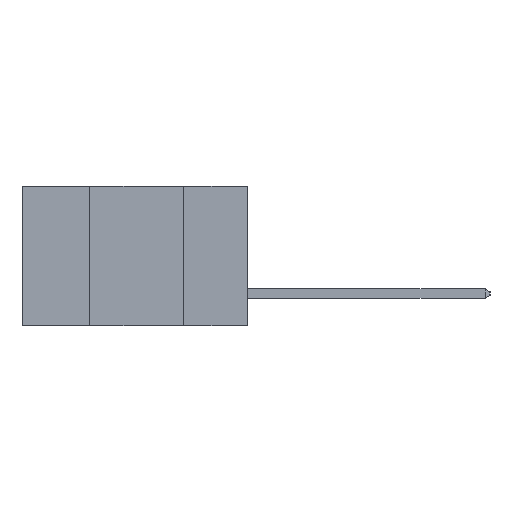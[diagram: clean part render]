
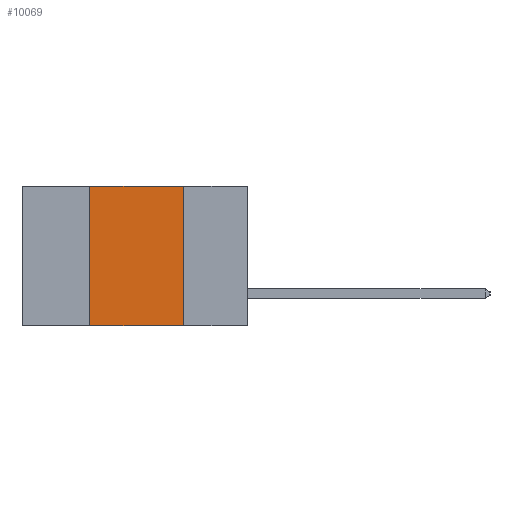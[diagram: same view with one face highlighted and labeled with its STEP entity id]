
A CAD part, left-side view. The second image highlights one B-rep face of the part: STEP entity #10069.
In plain terms, the highlighted planar face has unit normal (-1, 0, 0).
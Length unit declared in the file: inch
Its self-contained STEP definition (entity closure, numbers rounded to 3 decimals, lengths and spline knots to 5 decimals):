
#103 = CARTESIAN_POINT ( 'NONE',  ( 0., 0.6, 0. ) ) ;
#290 = ORIENTED_EDGE ( 'NONE', *, *, #16591, .T. ) ;
#345 = VERTEX_POINT ( 'NONE', #14618 ) ;
#537 = CARTESIAN_POINT ( 'NONE',  ( 0., 0.17, 0. ) ) ;
#634 = DIRECTION ( 'NONE',  ( 0., -1., 0. ) ) ;
#796 = LINE ( 'NONE', #537, #7163 ) ;
#844 = EDGE_CURVE ( 'NONE', #16369, #345, #12336, .T. ) ;
#1399 = DIRECTION ( 'NONE',  ( 0., 0., -1. ) ) ;
#2545 = EDGE_CURVE ( 'NONE', #10721, #10477, #796, .T. ) ;
#3326 = CARTESIAN_POINT ( 'NONE',  ( 0., 0.42, -0.37 ) ) ;
#4299 = LINE ( 'NONE', #103, #4698 ) ;
#4627 = ORIENTED_EDGE ( 'NONE', *, *, #4993, .F. ) ;
#4651 = ORIENTED_EDGE ( 'NONE', *, *, #2545, .F. ) ;
#4698 = VECTOR ( 'NONE', #634, 39.37008 ) ;
#4812 = EDGE_LOOP ( 'NONE', ( #4651, #4627, #12950, #290 ) ) ;
#4846 = CARTESIAN_POINT ( 'NONE',  ( 0., 0.6, 0. ) ) ;
#4993 = EDGE_CURVE ( 'NONE', #345, #10721, #4299, .T. ) ;
#5405 = VECTOR ( 'NONE', #6793, 39.37008 ) ;
#6147 = DIRECTION ( 'NONE',  ( 0., 0., -1. ) ) ;
#6793 = DIRECTION ( 'NONE',  ( 0., 0., 1. ) ) ;
#7163 = VECTOR ( 'NONE', #1399, 39.37008 ) ;
#7377 = VECTOR ( 'NONE', #7618, 39.37008 ) ;
#7618 = DIRECTION ( 'NONE',  ( 0., -1., 0. ) ) ;
#9984 = PLANE ( 'NONE',  #11144 ) ;
#10069 = ADVANCED_FACE ( 'NONE', ( #10407 ), #9984, .F. ) ;
#10407 = FACE_OUTER_BOUND ( 'NONE', #4812, .T. ) ;
#10477 = VERTEX_POINT ( 'NONE', #12062 ) ;
#10721 = VERTEX_POINT ( 'NONE', #13779 ) ;
#10831 = LINE ( 'NONE', #15340, #7377 ) ;
#11144 = AXIS2_PLACEMENT_3D ( 'NONE', #4846, #13901, #6147 ) ;
#12062 = CARTESIAN_POINT ( 'NONE',  ( 0., 0.17, -0.37 ) ) ;
#12336 = LINE ( 'NONE', #12603, #5405 ) ;
#12603 = CARTESIAN_POINT ( 'NONE',  ( 0., 0.42, 0. ) ) ;
#12950 = ORIENTED_EDGE ( 'NONE', *, *, #844, .F. ) ;
#13779 = CARTESIAN_POINT ( 'NONE',  ( 0., 0.17, 0. ) ) ;
#13901 = DIRECTION ( 'NONE',  ( 1., 0., 0. ) ) ;
#14618 = CARTESIAN_POINT ( 'NONE',  ( 0., 0.42, 0. ) ) ;
#15340 = CARTESIAN_POINT ( 'NONE',  ( 0., 0.6, -0.37 ) ) ;
#16369 = VERTEX_POINT ( 'NONE', #3326 ) ;
#16591 = EDGE_CURVE ( 'NONE', #16369, #10477, #10831, .T. ) ;
